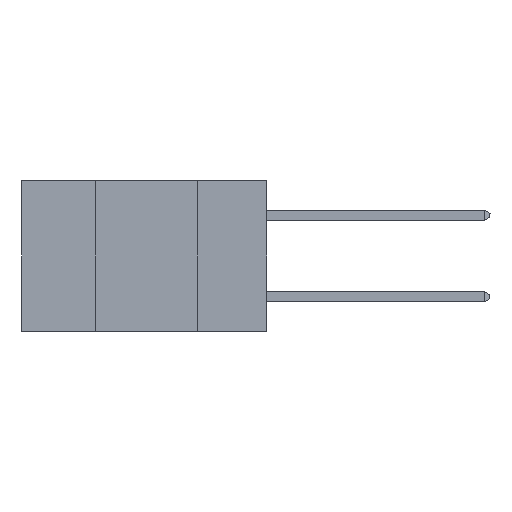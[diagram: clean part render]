
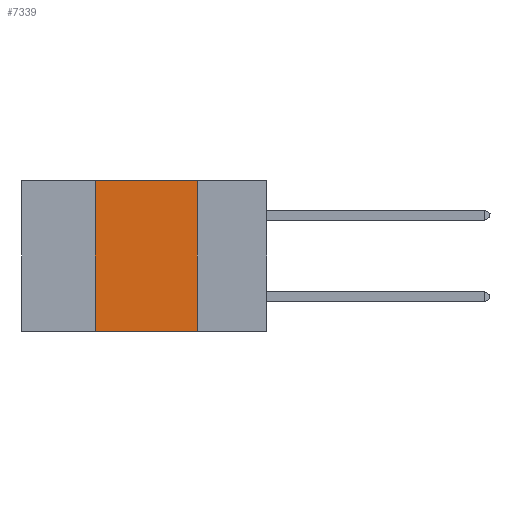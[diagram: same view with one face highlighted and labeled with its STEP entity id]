
A CAD part, left-side view. The second image highlights one B-rep face of the part: STEP entity #7339.
In plain terms, the highlighted planar face has unit normal (-1, 0, 0).
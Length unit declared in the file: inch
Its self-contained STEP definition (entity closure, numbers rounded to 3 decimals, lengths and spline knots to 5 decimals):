
#1785 = CARTESIAN_POINT ( 'NONE',  ( 0., 0.6, 0. ) ) ;
#3672 = CARTESIAN_POINT ( 'NONE',  ( 0., 0.17, 0. ) ) ;
#5481 = CARTESIAN_POINT ( 'NONE',  ( 0., 0.6, -0.37 ) ) ;
#5592 = LINE ( 'NONE', #35856, #8077 ) ;
#6028 = DIRECTION ( 'NONE',  ( 0., 0., -1. ) ) ;
#6815 = VERTEX_POINT ( 'NONE', #3672 ) ;
#7339 = ADVANCED_FACE ( 'NONE', ( #42346 ), #14930, .F. ) ;
#8043 = DIRECTION ( 'NONE',  ( 0., 0., 1. ) ) ;
#8077 = VECTOR ( 'NONE', #6028, 39.37008 ) ;
#12014 = AXIS2_PLACEMENT_3D ( 'NONE', #1785, #32250, #28968 ) ;
#14930 = PLANE ( 'NONE',  #12014 ) ;
#15149 = VECTOR ( 'NONE', #22573, 39.37008 ) ;
#16104 = DIRECTION ( 'NONE',  ( 0., -1., 0. ) ) ;
#17859 = EDGE_LOOP ( 'NONE', ( #24800, #28162, #36420, #31897 ) ) ;
#18629 = CARTESIAN_POINT ( 'NONE',  ( 0., 0.42, -0.37 ) ) ;
#22573 = DIRECTION ( 'NONE',  ( 0., -1., 0. ) ) ;
#23809 = VECTOR ( 'NONE', #16104, 39.37008 ) ;
#24800 = ORIENTED_EDGE ( 'NONE', *, *, #41305, .F. ) ;
#27582 = CARTESIAN_POINT ( 'NONE',  ( 0., 0.42, 0. ) ) ;
#27954 = EDGE_CURVE ( 'NONE', #42765, #32299, #38086, .T. ) ;
#28162 = ORIENTED_EDGE ( 'NONE', *, *, #31534, .F. ) ;
#28968 = DIRECTION ( 'NONE',  ( 0., 0., -1. ) ) ;
#29486 = CARTESIAN_POINT ( 'NONE',  ( 0., 0.6, 0. ) ) ;
#30052 = VERTEX_POINT ( 'NONE', #32503 ) ;
#31534 = EDGE_CURVE ( 'NONE', #32299, #6815, #36730, .T. ) ;
#31897 = ORIENTED_EDGE ( 'NONE', *, *, #42772, .T. ) ;
#32250 = DIRECTION ( 'NONE',  ( 1., 0., 0. ) ) ;
#32299 = VERTEX_POINT ( 'NONE', #35267 ) ;
#32503 = CARTESIAN_POINT ( 'NONE',  ( 0., 0.17, -0.37 ) ) ;
#35267 = CARTESIAN_POINT ( 'NONE',  ( 0., 0.42, 0. ) ) ;
#35529 = LINE ( 'NONE', #5481, #15149 ) ;
#35856 = CARTESIAN_POINT ( 'NONE',  ( 0., 0.17, 0. ) ) ;
#36420 = ORIENTED_EDGE ( 'NONE', *, *, #27954, .F. ) ;
#36730 = LINE ( 'NONE', #29486, #23809 ) ;
#38086 = LINE ( 'NONE', #27582, #42163 ) ;
#41305 = EDGE_CURVE ( 'NONE', #6815, #30052, #5592, .T. ) ;
#42163 = VECTOR ( 'NONE', #8043, 39.37008 ) ;
#42346 = FACE_OUTER_BOUND ( 'NONE', #17859, .T. ) ;
#42765 = VERTEX_POINT ( 'NONE', #18629 ) ;
#42772 = EDGE_CURVE ( 'NONE', #42765, #30052, #35529, .T. ) ;
